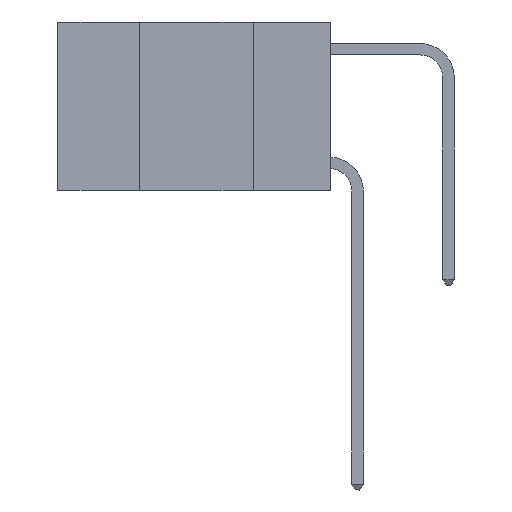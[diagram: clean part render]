
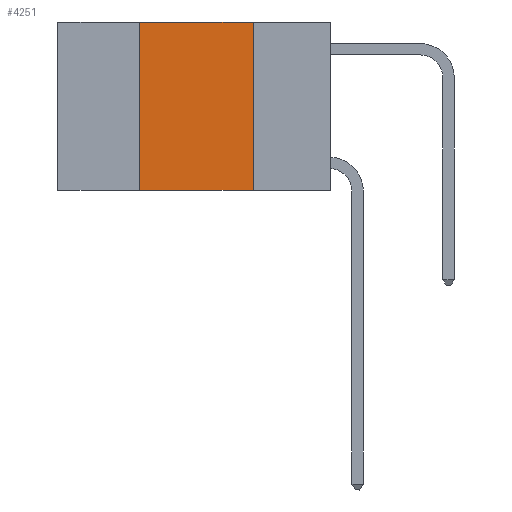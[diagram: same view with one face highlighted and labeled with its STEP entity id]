
A CAD part, left-side view. The second image highlights one B-rep face of the part: STEP entity #4251.
In plain terms, the highlighted planar face has unit normal (-1, 0, 0).
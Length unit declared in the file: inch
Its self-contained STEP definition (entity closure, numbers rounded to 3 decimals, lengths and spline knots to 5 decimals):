
#467 = LINE ( 'NONE', #9782, #10314 ) ;
#605 = ORIENTED_EDGE ( 'NONE', *, *, #11194, .T. ) ;
#672 = EDGE_CURVE ( 'NONE', #12978, #11250, #467, .T. ) ;
#742 = CARTESIAN_POINT ( 'NONE',  ( 0., 0.17, 0. ) ) ;
#749 = DIRECTION ( 'NONE',  ( 0., 0., -1. ) ) ;
#773 = ORIENTED_EDGE ( 'NONE', *, *, #12520, .F. ) ;
#1004 = DIRECTION ( 'NONE',  ( 0., -1., 0. ) ) ;
#1431 = ORIENTED_EDGE ( 'NONE', *, *, #9377, .F. ) ;
#2088 = VECTOR ( 'NONE', #4611, 39.37008 ) ;
#2404 = LINE ( 'NONE', #7635, #2088 ) ;
#2813 = VECTOR ( 'NONE', #749, 39.37008 ) ;
#2910 = DIRECTION ( 'NONE',  ( 1., 0., 0. ) ) ;
#2953 = VERTEX_POINT ( 'NONE', #6929 ) ;
#2988 = LINE ( 'NONE', #6920, #8130 ) ;
#3125 = CARTESIAN_POINT ( 'NONE',  ( 0., 0.17, -0.37 ) ) ;
#3397 = CARTESIAN_POINT ( 'NONE',  ( 0., 0.42, 0. ) ) ;
#4251 = ADVANCED_FACE ( 'NONE', ( #8559 ), #11957, .F. ) ;
#4460 = AXIS2_PLACEMENT_3D ( 'NONE', #5035, #2910, #10012 ) ;
#4611 = DIRECTION ( 'NONE',  ( 0., 0., 1. ) ) ;
#5035 = CARTESIAN_POINT ( 'NONE',  ( 0., 0.6, 0. ) ) ;
#5960 = VERTEX_POINT ( 'NONE', #3125 ) ;
#6920 = CARTESIAN_POINT ( 'NONE',  ( 0., 0.6, -0.37 ) ) ;
#6929 = CARTESIAN_POINT ( 'NONE',  ( 0., 0.42, -0.37 ) ) ;
#7635 = CARTESIAN_POINT ( 'NONE',  ( 0., 0.42, 0. ) ) ;
#7639 = EDGE_LOOP ( 'NONE', ( #773, #11556, #1431, #605 ) ) ;
#7851 = DIRECTION ( 'NONE',  ( 0., -1., 0. ) ) ;
#7902 = CARTESIAN_POINT ( 'NONE',  ( 0., 0.17, 0. ) ) ;
#8130 = VECTOR ( 'NONE', #7851, 39.37008 ) ;
#8262 = LINE ( 'NONE', #7902, #2813 ) ;
#8559 = FACE_OUTER_BOUND ( 'NONE', #7639, .T. ) ;
#9377 = EDGE_CURVE ( 'NONE', #2953, #12978, #2404, .T. ) ;
#9782 = CARTESIAN_POINT ( 'NONE',  ( 0., 0.6, 0. ) ) ;
#10012 = DIRECTION ( 'NONE',  ( 0., 0., -1. ) ) ;
#10314 = VECTOR ( 'NONE', #1004, 39.37008 ) ;
#11194 = EDGE_CURVE ( 'NONE', #2953, #5960, #2988, .T. ) ;
#11250 = VERTEX_POINT ( 'NONE', #742 ) ;
#11556 = ORIENTED_EDGE ( 'NONE', *, *, #672, .F. ) ;
#11957 = PLANE ( 'NONE',  #4460 ) ;
#12520 = EDGE_CURVE ( 'NONE', #11250, #5960, #8262, .T. ) ;
#12978 = VERTEX_POINT ( 'NONE', #3397 ) ;
